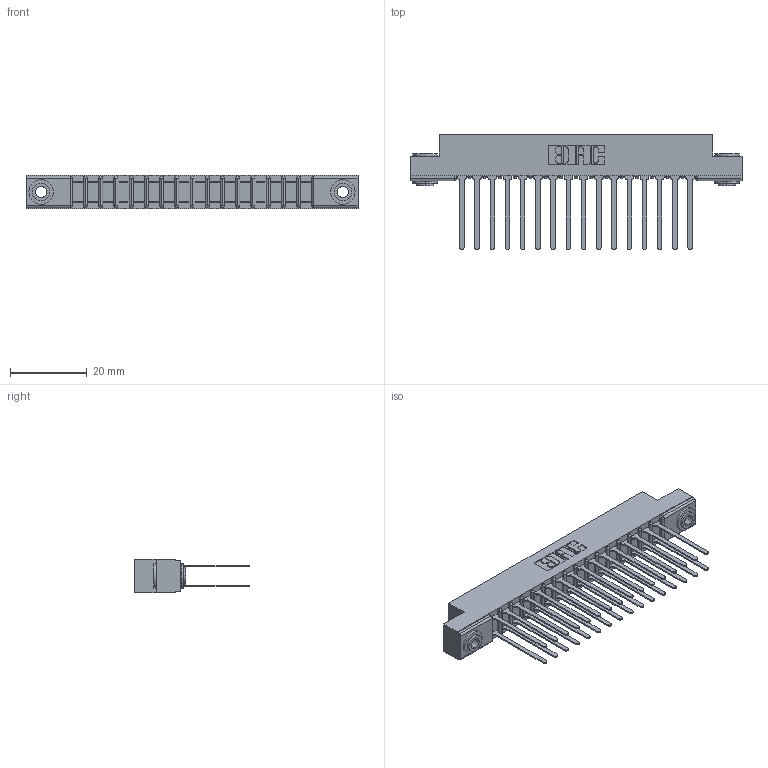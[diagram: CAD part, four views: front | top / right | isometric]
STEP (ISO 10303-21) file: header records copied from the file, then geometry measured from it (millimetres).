
FILE_DESCRIPTION (( 'STEP AP203' ), '1' );
FILE_NAME ('307-032-440-203.STEP', '2020-09-29T11:01:44', ( '' ), ( '' ), 'SwSTEP 2.0', 'SolidWorks 2020', '' );
FILE_SCHEMA (( 'CONFIG_CONTROL_DESIGN' ));
Length unit declared in the file: inch
Products named in the file (4): 307-032-440-203; 307-290-001_540; 307 Part_.156 Dia Mounting Holes; 345-250-002_345-250-002-102
Assembly tree (35 placements, depth 2):
  307-032-440-203
    307 Part_.156 Dia Mounting Holes
    307-290-001_540  x32
    345-250-002_345-250-002-102  x2
Bounding box: 86.41 x 30 x 8.71 mm (x, y, z)
Volume: 5832.8 mm3; surface area: 11256.2 mm2
Topology: 35 solids, 35 shells, 1659 faces, 4595 edges, 2970 vertices
Faces by surface type: plane 1086, cylinder 531, sphere 34, cone 8
Entity records: 18467 total; most frequent: CARTESIAN_POINT 3009, DIRECTION 2973, ORIENTED_EDGE 2970, EDGE_CURVE 1485, LINE 1121, VECTOR 1121, VERTEX_POINT 962, AXIS2_PLACEMENT_3D 926
